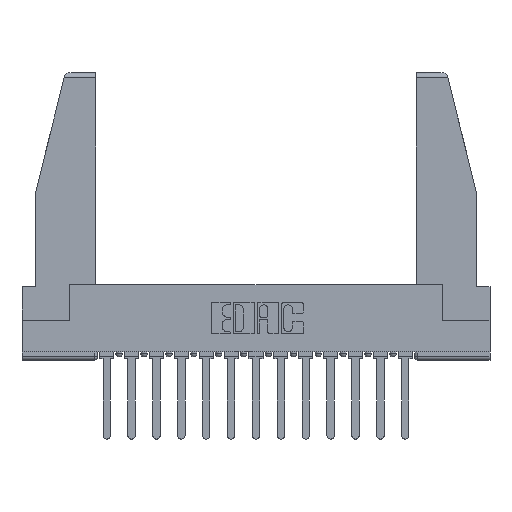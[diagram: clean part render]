
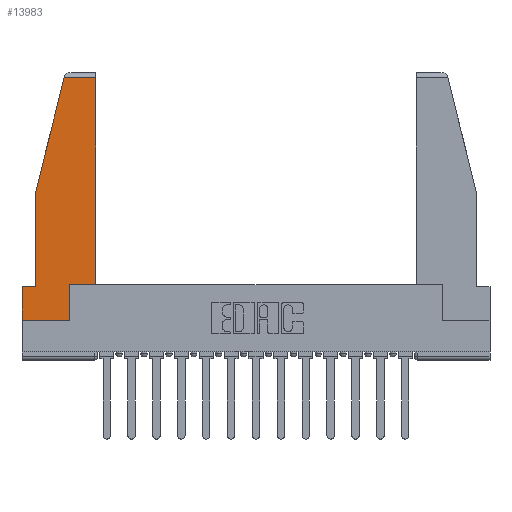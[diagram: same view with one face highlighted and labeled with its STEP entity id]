
A CAD part, top view. The second image highlights one B-rep face of the part: STEP entity #13983.
In plain terms, the highlighted planar face has unit normal (0, 0, 1).
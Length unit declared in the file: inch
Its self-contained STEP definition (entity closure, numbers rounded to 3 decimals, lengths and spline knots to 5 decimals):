
#43 = CARTESIAN_POINT ( 'NONE',  ( 0., 0.21, 0. ) ) ;
#639 = CARTESIAN_POINT ( 'NONE',  ( 0.271, 1.55, 0. ) ) ;
#660 = VERTEX_POINT ( 'NONE', #11989 ) ;
#1033 = EDGE_CURVE ( 'NONE', #16898, #660, #2993, .T. ) ;
#1096 = ORIENTED_EDGE ( 'NONE', *, *, #14380, .T. ) ;
#1592 = ORIENTED_EDGE ( 'NONE', *, *, #7754, .T. ) ;
#2216 = CARTESIAN_POINT ( 'NONE',  ( 0.461, 0.223, 0. ) ) ;
#2272 = VECTOR ( 'NONE', #7790, 39.37008 ) ;
#2336 = CARTESIAN_POINT ( 'NONE',  ( 0.297, 0., 0. ) ) ;
#2434 = EDGE_LOOP ( 'NONE', ( #5179, #4483, #10789, #12747, #12548, #1592, #6067, #5956, #1096 ) ) ;
#2494 = DIRECTION ( 'NONE',  ( 1., 0., 0. ) ) ;
#2647 = LINE ( 'NONE', #3404, #8234 ) ;
#2705 = LINE ( 'NONE', #2216, #17816 ) ;
#2900 = EDGE_CURVE ( 'NONE', #3697, #5617, #2705, .T. ) ;
#2993 = LINE ( 'NONE', #639, #16810 ) ;
#3089 = VERTEX_POINT ( 'NONE', #4060 ) ;
#3404 = CARTESIAN_POINT ( 'NONE',  ( 0.086, 0.8, 0. ) ) ;
#3432 = DIRECTION ( 'NONE',  ( -0.239, -0.971, 0. ) ) ;
#3503 = VERTEX_POINT ( 'NONE', #17397 ) ;
#3697 = VERTEX_POINT ( 'NONE', #4270 ) ;
#3943 = DIRECTION ( 'NONE',  ( 1., 0., 0. ) ) ;
#4017 = LINE ( 'NONE', #43, #14351 ) ;
#4060 = CARTESIAN_POINT ( 'NONE',  ( 0.297, 0., 0. ) ) ;
#4270 = CARTESIAN_POINT ( 'NONE',  ( 0.461, 0.223, 0. ) ) ;
#4483 = ORIENTED_EDGE ( 'NONE', *, *, #6985, .T. ) ;
#5179 = ORIENTED_EDGE ( 'NONE', *, *, #2900, .T. ) ;
#5617 = VERTEX_POINT ( 'NONE', #9632 ) ;
#5640 = DIRECTION ( 'NONE',  ( 0., -1., 0. ) ) ;
#5956 = ORIENTED_EDGE ( 'NONE', *, *, #6802, .T. ) ;
#6067 = ORIENTED_EDGE ( 'NONE', *, *, #11077, .T. ) ;
#6215 = VECTOR ( 'NONE', #17527, 39.37008 ) ;
#6442 = CARTESIAN_POINT ( 'NONE',  ( 0., 0.21, 0. ) ) ;
#6802 = EDGE_CURVE ( 'NONE', #3089, #9897, #16797, .T. ) ;
#6837 = CARTESIAN_POINT ( 'NONE',  ( 0., 0., 0. ) ) ;
#6985 = EDGE_CURVE ( 'NONE', #5617, #16898, #14822, .T. ) ;
#7364 = DIRECTION ( 'NONE',  ( 0., -1., 0. ) ) ;
#7434 = FACE_OUTER_BOUND ( 'NONE', #2434, .T. ) ;
#7754 = EDGE_CURVE ( 'NONE', #13231, #3503, #17206, .T. ) ;
#7790 = DIRECTION ( 'NONE',  ( 1., 0., 0. ) ) ;
#7970 = CARTESIAN_POINT ( 'NONE',  ( 0., 1.52, 0. ) ) ;
#8234 = VECTOR ( 'NONE', #7364, 39.37008 ) ;
#8299 = DIRECTION ( 'NONE',  ( -1., 0., 0. ) ) ;
#9371 = LINE ( 'NONE', #11766, #2272 ) ;
#9632 = CARTESIAN_POINT ( 'NONE',  ( 0.461, 1.52, 0. ) ) ;
#9821 = VECTOR ( 'NONE', #5640, 39.37008 ) ;
#9897 = VERTEX_POINT ( 'NONE', #17444 ) ;
#10193 = AXIS2_PLACEMENT_3D ( 'NONE', #6837, #11088, #3943 ) ;
#10194 = VECTOR ( 'NONE', #2494, 39.37008 ) ;
#10704 = VECTOR ( 'NONE', #15029, 39.37008 ) ;
#10789 = ORIENTED_EDGE ( 'NONE', *, *, #1033, .T. ) ;
#11077 = EDGE_CURVE ( 'NONE', #3503, #3089, #17561, .T. ) ;
#11088 = DIRECTION ( 'NONE',  ( 0., 0., 1. ) ) ;
#11766 = CARTESIAN_POINT ( 'NONE',  ( 0.297, 0.223, 0. ) ) ;
#11834 = DIRECTION ( 'NONE',  ( 0., 1., 0. ) ) ;
#11989 = CARTESIAN_POINT ( 'NONE',  ( 0.086, 0.8, 0. ) ) ;
#12295 = CARTESIAN_POINT ( 'NONE',  ( 0., 0., 0. ) ) ;
#12548 = ORIENTED_EDGE ( 'NONE', *, *, #13470, .T. ) ;
#12747 = ORIENTED_EDGE ( 'NONE', *, *, #16369, .T. ) ;
#13231 = VERTEX_POINT ( 'NONE', #6442 ) ;
#13470 = EDGE_CURVE ( 'NONE', #13657, #13231, #4017, .T. ) ;
#13657 = VERTEX_POINT ( 'NONE', #15778 ) ;
#13983 = ADVANCED_FACE ( 'NONE', ( #7434 ), #16508, .T. ) ;
#14062 = CARTESIAN_POINT ( 'NONE',  ( 0., 0.21, 0. ) ) ;
#14351 = VECTOR ( 'NONE', #8299, 39.37008 ) ;
#14380 = EDGE_CURVE ( 'NONE', #9897, #3697, #9371, .T. ) ;
#14822 = LINE ( 'NONE', #7970, #10704 ) ;
#15029 = DIRECTION ( 'NONE',  ( -1., 0., 0. ) ) ;
#15778 = CARTESIAN_POINT ( 'NONE',  ( 0.086, 0.21, 0. ) ) ;
#16369 = EDGE_CURVE ( 'NONE', #660, #13657, #2647, .T. ) ;
#16508 = PLANE ( 'NONE',  #10193 ) ;
#16797 = LINE ( 'NONE', #2336, #6215 ) ;
#16810 = VECTOR ( 'NONE', #3432, 39.37008 ) ;
#16898 = VERTEX_POINT ( 'NONE', #16967 ) ;
#16967 = CARTESIAN_POINT ( 'NONE',  ( 0.2636, 1.52, 0. ) ) ;
#17206 = LINE ( 'NONE', #14062, #9821 ) ;
#17397 = CARTESIAN_POINT ( 'NONE',  ( 0., 0., 0. ) ) ;
#17444 = CARTESIAN_POINT ( 'NONE',  ( 0.297, 0.223, 0. ) ) ;
#17527 = DIRECTION ( 'NONE',  ( 0., 1., 0. ) ) ;
#17561 = LINE ( 'NONE', #12295, #10194 ) ;
#17816 = VECTOR ( 'NONE', #11834, 39.37008 ) ;
